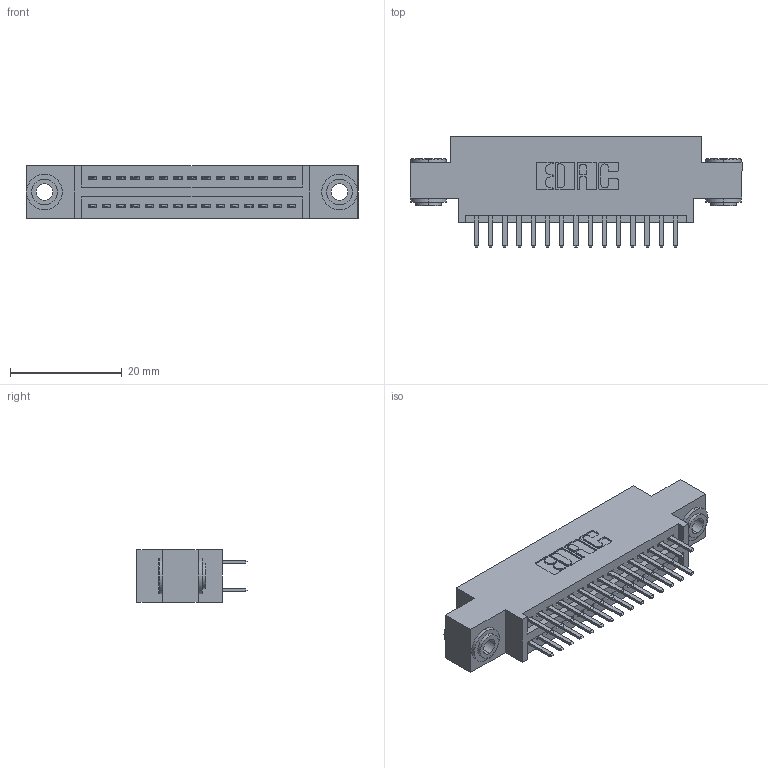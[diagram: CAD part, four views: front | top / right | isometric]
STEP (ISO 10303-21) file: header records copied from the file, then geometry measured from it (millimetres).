
FILE_DESCRIPTION (( 'STEP AP203' ), '1' );
FILE_NAME ('395-030-520-803.STEP', '2018-11-10T23:13:11', ( '' ), ( '' ), 'SwSTEP 2.0', 'SolidWorks 2016', '' );
FILE_SCHEMA (( 'CONFIG_CONTROL_DESIGN' ));
Length unit declared in the file: inch
Products named in the file (4): 345 Part_0.170 Offset - 0.156 Dia-TH; 345-250-002_345-250-002-102; 345-292-001_345-293-120; 395-030-520-803
Assembly tree (33 placements, depth 2):
  395-030-520-803
    345 Part_0.170 Offset - 0.156 Dia-TH
    345-292-001_345-293-120  x30
    345-250-002_345-250-002-102  x2
Bounding box: 59.31 x 19.68 x 9.4 mm (x, y, z)
Volume: 5403.5 mm3; surface area: 7784.7 mm2
Topology: 33 solids, 33 shells, 1788 faces, 5139 edges, 3342 vertices
Faces by surface type: plane 1144, cylinder 636, cone 8
Entity records: 16300 total; most frequent: CARTESIAN_POINT 2747, ORIENTED_EDGE 2662, DIRECTION 2473, EDGE_CURVE 1331, LINE 1111, VECTOR 1111, VERTEX_POINT 882, AXIS2_PLACEMENT_3D 681
